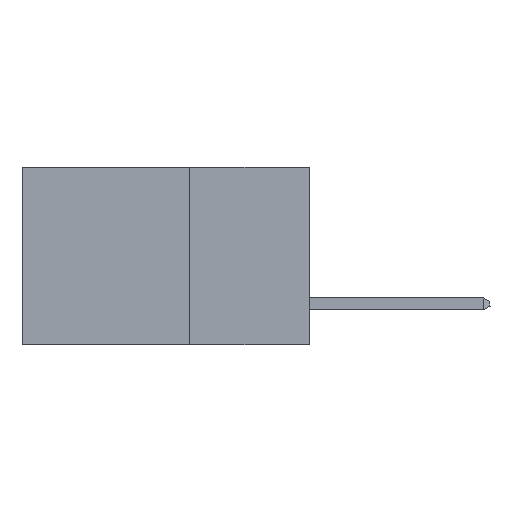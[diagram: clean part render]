
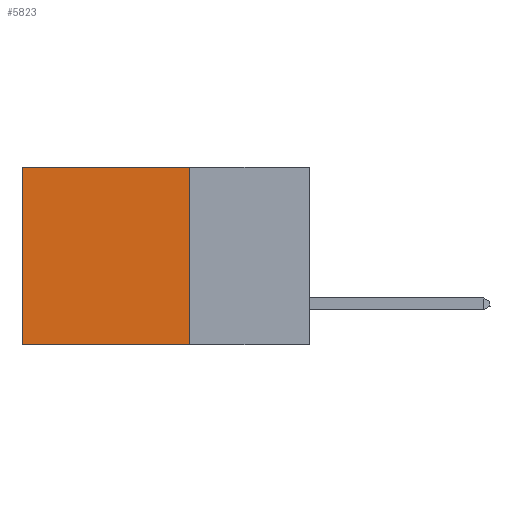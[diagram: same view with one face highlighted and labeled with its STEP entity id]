
A CAD part, left-side view. The second image highlights one B-rep face of the part: STEP entity #5823.
In plain terms, the highlighted planar face has unit normal (-1, 0, 0).
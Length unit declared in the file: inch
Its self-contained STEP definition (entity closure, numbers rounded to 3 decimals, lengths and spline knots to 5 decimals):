
#1681 = VERTEX_POINT ( 'NONE', #35523 ) ;
#2066 = CARTESIAN_POINT ( 'NONE',  ( 0.2875, 0.25, 0. ) ) ;
#2730 = CARTESIAN_POINT ( 'NONE',  ( 0.2875, 0.6, -0.37 ) ) ;
#4105 = VECTOR ( 'NONE', #22248, 39.37008 ) ;
#4507 = EDGE_CURVE ( 'NONE', #29307, #15933, #21212, .T. ) ;
#4680 = CARTESIAN_POINT ( 'NONE',  ( 0.2875, 0.25, -0.37 ) ) ;
#5067 = EDGE_LOOP ( 'NONE', ( #8399, #13434, #33743, #29927 ) ) ;
#5599 = EDGE_CURVE ( 'NONE', #1681, #29307, #20688, .T. ) ;
#5625 = CARTESIAN_POINT ( 'NONE',  ( 0.2875, 0.6, 0. ) ) ;
#5740 = FACE_OUTER_BOUND ( 'NONE', #5067, .T. ) ;
#5823 = ADVANCED_FACE ( 'NONE', ( #5740 ), #11863, .F. ) ;
#6736 = EDGE_CURVE ( 'NONE', #7368, #15933, #17466, .T. ) ;
#7368 = VERTEX_POINT ( 'NONE', #33396 ) ;
#8399 = ORIENTED_EDGE ( 'NONE', *, *, #4507, .T. ) ;
#9377 = AXIS2_PLACEMENT_3D ( 'NONE', #26123, #31893, #14770 ) ;
#9748 = EDGE_CURVE ( 'NONE', #1681, #7368, #18656, .T. ) ;
#10555 = DIRECTION ( 'NONE',  ( 0., 1., 0. ) ) ;
#11863 = PLANE ( 'NONE',  #9377 ) ;
#13434 = ORIENTED_EDGE ( 'NONE', *, *, #6736, .F. ) ;
#13964 = VECTOR ( 'NONE', #16810, 39.37008 ) ;
#14770 = DIRECTION ( 'NONE',  ( 0., 0., -1. ) ) ;
#15933 = VERTEX_POINT ( 'NONE', #2730 ) ;
#16810 = DIRECTION ( 'NONE',  ( 0., 1., 0. ) ) ;
#17466 = LINE ( 'NONE', #4680, #32633 ) ;
#18656 = LINE ( 'NONE', #2066, #4105 ) ;
#20688 = LINE ( 'NONE', #33858, #13964 ) ;
#21212 = LINE ( 'NONE', #5625, #35445 ) ;
#22248 = DIRECTION ( 'NONE',  ( 0., 0., -1. ) ) ;
#25770 = DIRECTION ( 'NONE',  ( 0., 0., -1. ) ) ;
#26123 = CARTESIAN_POINT ( 'NONE',  ( 0.2875, 0.25, 0. ) ) ;
#29307 = VERTEX_POINT ( 'NONE', #30097 ) ;
#29927 = ORIENTED_EDGE ( 'NONE', *, *, #5599, .T. ) ;
#30097 = CARTESIAN_POINT ( 'NONE',  ( 0.2875, 0.6, 0. ) ) ;
#31893 = DIRECTION ( 'NONE',  ( 1., 0., 0. ) ) ;
#32633 = VECTOR ( 'NONE', #10555, 39.37008 ) ;
#33396 = CARTESIAN_POINT ( 'NONE',  ( 0.2875, 0.25, -0.37 ) ) ;
#33743 = ORIENTED_EDGE ( 'NONE', *, *, #9748, .F. ) ;
#33858 = CARTESIAN_POINT ( 'NONE',  ( 0.2875, 0.25, 0. ) ) ;
#35445 = VECTOR ( 'NONE', #25770, 39.37008 ) ;
#35523 = CARTESIAN_POINT ( 'NONE',  ( 0.2875, 0.25, 0. ) ) ;
